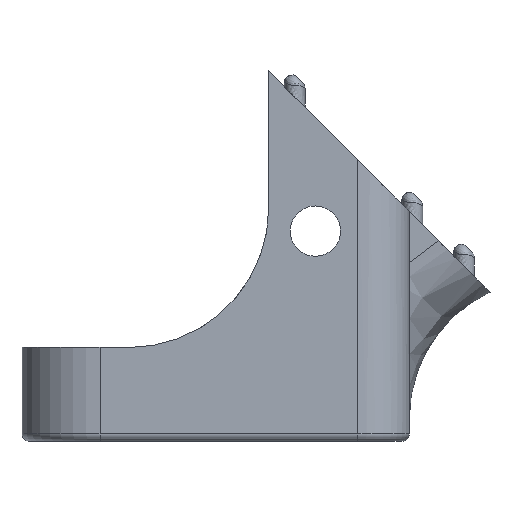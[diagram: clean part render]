
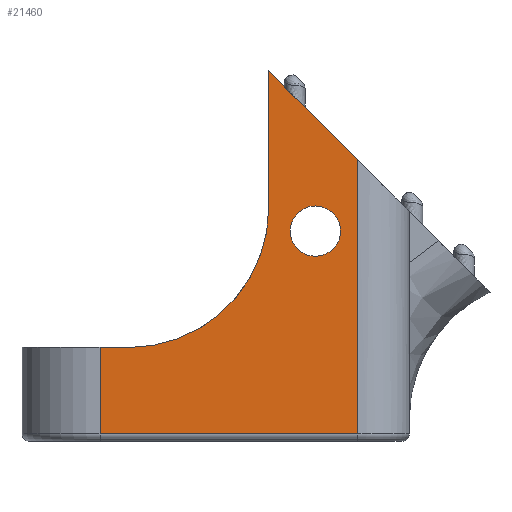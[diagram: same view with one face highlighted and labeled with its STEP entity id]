
A CAD part, front view. The second image highlights one B-rep face of the part: STEP entity #21460.
In plain terms, the highlighted planar face has unit normal (0, -1, 0).
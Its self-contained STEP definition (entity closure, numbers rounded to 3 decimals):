
#819 = CARTESIAN_POINT ( 'NONE',  ( 14.936, -20.754, 18.376 ) ) ;
#828 = CARTESIAN_POINT ( 'NONE',  ( 2.817, -20.754, 30.495 ) ) ;
#1117 = LINE ( 'NONE', #12061, #4231 ) ;
#1294 = LINE ( 'NONE', #24923, #20965 ) ;
#1994 = LINE ( 'NONE', #28354, #2030 ) ;
#2030 = VECTOR ( 'NONE', #5353, 1000. ) ;
#2221 = ORIENTED_EDGE ( 'NONE', *, *, #24448, .F. ) ;
#2352 = AXIS2_PLACEMENT_3D ( 'NONE', #20234, #4864, #22792 ) ;
#2448 = ORIENTED_EDGE ( 'NONE', *, *, #24258, .T. ) ;
#2633 = DIRECTION ( 'NONE',  ( 0., -1., 0. ) ) ;
#2960 = DIRECTION ( 'NONE',  ( 0., 0., -1. ) ) ;
#3825 = AXIS2_PLACEMENT_3D ( 'NONE', #17978, #2633, #20591 ) ;
#4079 = AXIS2_PLACEMENT_3D ( 'NONE', #12140, #29992, #14710 ) ;
#4231 = VECTOR ( 'NONE', #19833, 1000. ) ;
#4864 = DIRECTION ( 'NONE',  ( 0., -1., 0. ) ) ;
#4891 = LINE ( 'NONE', #23567, #24529 ) ;
#5170 = ORIENTED_EDGE ( 'NONE', *, *, #25500, .T. ) ;
#5353 = DIRECTION ( 'NONE',  ( 0., 0., 1. ) ) ;
#5434 = ORIENTED_EDGE ( 'NONE', *, *, #25441, .T. ) ;
#5543 = CARTESIAN_POINT ( 'NONE',  ( 14.936, -20.754, -7.238 ) ) ;
#5932 = AXIS2_PLACEMENT_3D ( 'NONE', #28475, #10822, #28683 ) ;
#6232 = CARTESIAN_POINT ( 'NONE',  ( -16.233, -20.754, -7.238 ) ) ;
#7002 = CARTESIAN_POINT ( 'NONE',  ( 2.817, -20.754, 11.812 ) ) ;
#8258 = PLANE ( 'NONE',  #5932 ) ;
#8370 = VERTEX_POINT ( 'NONE', #14364 ) ;
#8434 = VERTEX_POINT ( 'NONE', #26864 ) ;
#8885 = CARTESIAN_POINT ( 'NONE',  ( -20.199, -20.754, -7.238 ) ) ;
#9055 = ORIENTED_EDGE ( 'NONE', *, *, #25490, .T. ) ;
#10579 = CARTESIAN_POINT ( 'NONE',  ( -20.199, -20.754, 149.058 ) ) ;
#10789 = DIRECTION ( 'NONE',  ( 1., 0., 0. ) ) ;
#10822 = DIRECTION ( 'NONE',  ( 0., -1., 0. ) ) ;
#11696 = VECTOR ( 'NONE', #2960, 1000. ) ;
#12061 = CARTESIAN_POINT ( 'NONE',  ( -50.405, -20.754, 83.717 ) ) ;
#12140 = CARTESIAN_POINT ( 'NONE',  ( -16.233, -20.754, 11.812 ) ) ;
#13290 = LINE ( 'NONE', #5543, #25301 ) ;
#14046 = VERTEX_POINT ( 'NONE', #828 ) ;
#14089 = VERTEX_POINT ( 'NONE', #819 ) ;
#14271 = VERTEX_POINT ( 'NONE', #7002 ) ;
#14364 = CARTESIAN_POINT ( 'NONE',  ( 9.179, -20.754, 5.208 ) ) ;
#14561 = VERTEX_POINT ( 'NONE', #6232 ) ;
#14589 = VERTEX_POINT ( 'NONE', #8885 ) ;
#14617 = VERTEX_POINT ( 'NONE', #26929 ) ;
#14684 = VERTEX_POINT ( 'NONE', #29311 ) ;
#14710 = DIRECTION ( 'NONE',  ( 0., 0., 1. ) ) ;
#16543 = FACE_OUTER_BOUND ( 'NONE', #22450, .T. ) ;
#16789 = EDGE_CURVE ( 'NONE', #14684, #14089, #1994, .T. ) ;
#16858 = EDGE_LOOP ( 'NONE', ( #18289, #18448 ) ) ;
#17978 = CARTESIAN_POINT ( 'NONE',  ( 9.179, -20.754, 8.637 ) ) ;
#18083 = ORIENTED_EDGE ( 'NONE', *, *, #16789, .T. ) ;
#18289 = ORIENTED_EDGE ( 'NONE', *, *, #28400, .F. ) ;
#18448 = ORIENTED_EDGE ( 'NONE', *, *, #24792, .F. ) ;
#18532 = LINE ( 'NONE', #10579, #11696 ) ;
#19833 = DIRECTION ( 'NONE',  ( 0.707, 0., -0.707 ) ) ;
#20234 = CARTESIAN_POINT ( 'NONE',  ( 9.179, -20.754, 8.637 ) ) ;
#20591 = DIRECTION ( 'NONE',  ( 0., 0., 1. ) ) ;
#20658 = EDGE_CURVE ( 'NONE', #14046, #14089, #1117, .T. ) ;
#20965 = VECTOR ( 'NONE', #22468, 1000. ) ;
#21460 = ADVANCED_FACE ( 'NONE', ( #16543, #23372 ), #8258, .T. ) ;
#22450 = EDGE_LOOP ( 'NONE', ( #32797, #2221, #2448, #5170, #5434, #9055, #18083 ) ) ;
#22468 = DIRECTION ( 'NONE',  ( 0., 0., 1. ) ) ;
#22792 = DIRECTION ( 'NONE',  ( 0., 0., 1. ) ) ;
#23372 = FACE_BOUND ( 'NONE', #16858, .T. ) ;
#23567 = CARTESIAN_POINT ( 'NONE',  ( 14.936, -20.754, -19.014 ) ) ;
#24258 = EDGE_CURVE ( 'NONE', #14271, #14561, #29275, .T. ) ;
#24448 = EDGE_CURVE ( 'NONE', #14271, #14046, #1294, .T. ) ;
#24529 = VECTOR ( 'NONE', #10789, 1000. ) ;
#24792 = EDGE_CURVE ( 'NONE', #8370, #8434, #26907, .T. ) ;
#24923 = CARTESIAN_POINT ( 'NONE',  ( 2.817, -20.754, 170.562 ) ) ;
#25301 = VECTOR ( 'NONE', #31175, 1000. ) ;
#25441 = EDGE_CURVE ( 'NONE', #14589, #14617, #18532, .T. ) ;
#25490 = EDGE_CURVE ( 'NONE', #14617, #14684, #4891, .T. ) ;
#25500 = EDGE_CURVE ( 'NONE', #14561, #14589, #13290, .T. ) ;
#26864 = CARTESIAN_POINT ( 'NONE',  ( 9.179, -20.754, 12.066 ) ) ;
#26907 = CIRCLE ( 'NONE', #3825, 3.429 ) ;
#26929 = CARTESIAN_POINT ( 'NONE',  ( -20.199, -20.754, -19.014 ) ) ;
#27131 = CIRCLE ( 'NONE', #2352, 3.429 ) ;
#28354 = CARTESIAN_POINT ( 'NONE',  ( 14.936, -20.754, 149.058 ) ) ;
#28400 = EDGE_CURVE ( 'NONE', #8434, #8370, #27131, .T. ) ;
#28475 = CARTESIAN_POINT ( 'NONE',  ( 14.936, -20.754, 149.058 ) ) ;
#28683 = DIRECTION ( 'NONE',  ( 0., 0., 1. ) ) ;
#29275 = CIRCLE ( 'NONE', #4079, 19.05 ) ;
#29311 = CARTESIAN_POINT ( 'NONE',  ( 14.936, -20.754, -19.014 ) ) ;
#29992 = DIRECTION ( 'NONE',  ( 0., 1., 0. ) ) ;
#31175 = DIRECTION ( 'NONE',  ( -1., 0., 0. ) ) ;
#32797 = ORIENTED_EDGE ( 'NONE', *, *, #20658, .F. ) ;
